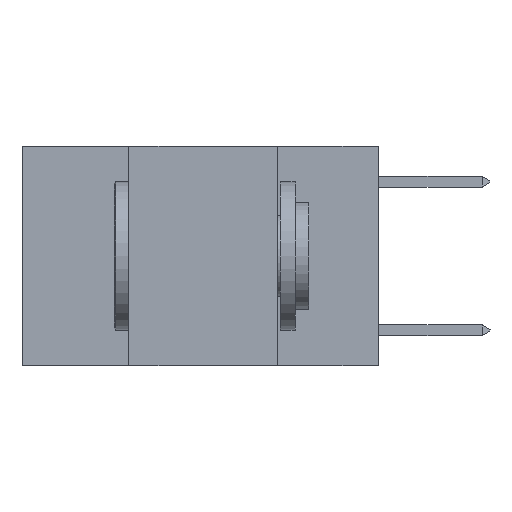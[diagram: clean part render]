
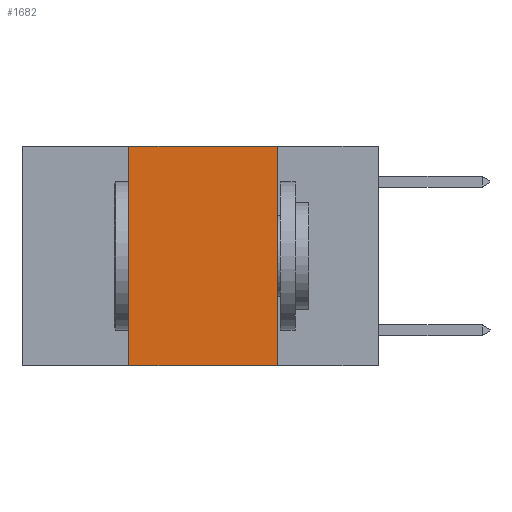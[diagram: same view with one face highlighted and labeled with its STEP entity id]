
A CAD part, left-side view. The second image highlights one B-rep face of the part: STEP entity #1682.
In plain terms, the highlighted planar face has unit normal (-1, 0, 0).
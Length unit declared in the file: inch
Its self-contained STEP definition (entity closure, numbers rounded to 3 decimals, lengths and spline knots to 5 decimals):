
#149 = VECTOR ( 'NONE', #729, 39.37008 ) ;
#696 = LINE ( 'NONE', #4990, #2703 ) ;
#729 = DIRECTION ( 'NONE',  ( 0., 0., 1. ) ) ;
#879 = LINE ( 'NONE', #6487, #2095 ) ;
#1443 = VERTEX_POINT ( 'NONE', #7339 ) ;
#1576 = EDGE_LOOP ( 'NONE', ( #6593, #6479, #6448, #6879 ) ) ;
#1682 = ADVANCED_FACE ( 'NONE', ( #3449 ), #5201, .F. ) ;
#2002 = DIRECTION ( 'NONE',  ( 0., -1., 0. ) ) ;
#2095 = VECTOR ( 'NONE', #7263, 39.37008 ) ;
#2226 = VECTOR ( 'NONE', #2002, 39.37008 ) ;
#2703 = VECTOR ( 'NONE', #5763, 39.37008 ) ;
#3322 = EDGE_CURVE ( 'NONE', #9772, #5942, #10108, .T. ) ;
#3449 = FACE_OUTER_BOUND ( 'NONE', #1576, .T. ) ;
#3583 = AXIS2_PLACEMENT_3D ( 'NONE', #5415, #4975, #4968 ) ;
#4347 = LINE ( 'NONE', #4393, #2226 ) ;
#4393 = CARTESIAN_POINT ( 'NONE',  ( 0., 0.6, 0. ) ) ;
#4505 = CARTESIAN_POINT ( 'NONE',  ( 0., 0.42, -0.37 ) ) ;
#4968 = DIRECTION ( 'NONE',  ( 0., 0., -1. ) ) ;
#4975 = DIRECTION ( 'NONE',  ( 1., 0., 0. ) ) ;
#4990 = CARTESIAN_POINT ( 'NONE',  ( 0., 0.17, 0. ) ) ;
#5201 = PLANE ( 'NONE',  #3583 ) ;
#5415 = CARTESIAN_POINT ( 'NONE',  ( 0., 0.6, 0. ) ) ;
#5763 = DIRECTION ( 'NONE',  ( 0., 0., -1. ) ) ;
#5942 = VERTEX_POINT ( 'NONE', #8815 ) ;
#6448 = ORIENTED_EDGE ( 'NONE', *, *, #3322, .F. ) ;
#6479 = ORIENTED_EDGE ( 'NONE', *, *, #7670, .F. ) ;
#6487 = CARTESIAN_POINT ( 'NONE',  ( 0., 0.6, -0.37 ) ) ;
#6592 = EDGE_CURVE ( 'NONE', #9772, #1443, #879, .T. ) ;
#6593 = ORIENTED_EDGE ( 'NONE', *, *, #9517, .F. ) ;
#6789 = CARTESIAN_POINT ( 'NONE',  ( 0., 0.17, 0. ) ) ;
#6879 = ORIENTED_EDGE ( 'NONE', *, *, #6592, .T. ) ;
#7263 = DIRECTION ( 'NONE',  ( 0., -1., 0. ) ) ;
#7339 = CARTESIAN_POINT ( 'NONE',  ( 0., 0.17, -0.37 ) ) ;
#7670 = EDGE_CURVE ( 'NONE', #5942, #9244, #4347, .T. ) ;
#8498 = CARTESIAN_POINT ( 'NONE',  ( 0., 0.42, 0. ) ) ;
#8815 = CARTESIAN_POINT ( 'NONE',  ( 0., 0.42, 0. ) ) ;
#9244 = VERTEX_POINT ( 'NONE', #6789 ) ;
#9517 = EDGE_CURVE ( 'NONE', #9244, #1443, #696, .T. ) ;
#9772 = VERTEX_POINT ( 'NONE', #4505 ) ;
#10108 = LINE ( 'NONE', #8498, #149 ) ;
